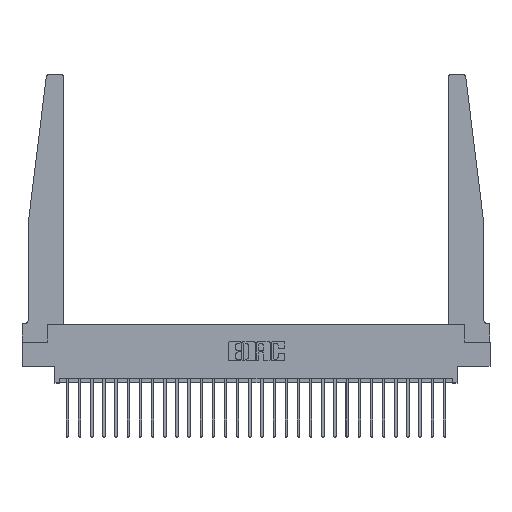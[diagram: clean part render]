
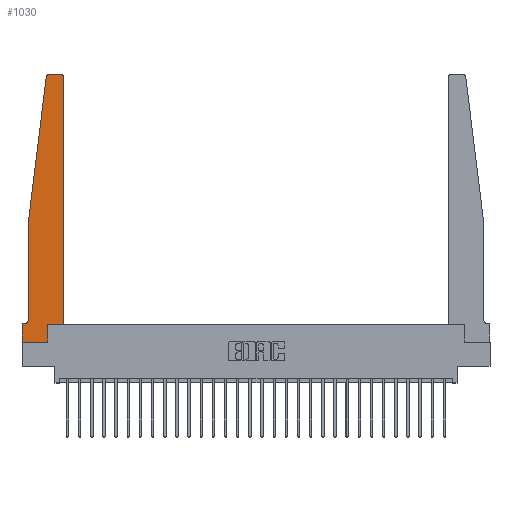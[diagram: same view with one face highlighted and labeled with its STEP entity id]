
A CAD part, top view. The second image highlights one B-rep face of the part: STEP entity #1030.
In plain terms, the highlighted planar face has unit normal (0, 0, 1).
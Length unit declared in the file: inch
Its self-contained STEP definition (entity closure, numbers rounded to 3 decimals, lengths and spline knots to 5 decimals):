
#141 = DIRECTION ( 'NONE',  ( -0.122, -0.992, 0. ) ) ;
#332 = DIRECTION ( 'NONE',  ( 1., 0., 0. ) ) ;
#891 = CARTESIAN_POINT ( 'NONE',  ( 0., 0., 0.37 ) ) ;
#1030 = ADVANCED_FACE ( 'NONE', ( #24861 ), #23354, .T. ) ;
#1106 = CIRCLE ( 'NONE', #11895, 0.03 ) ;
#1313 = VERTEX_POINT ( 'NONE', #19991 ) ;
#1432 = CARTESIAN_POINT ( 'NONE',  ( 0.2605, 0.18, 0.37 ) ) ;
#1592 = LINE ( 'NONE', #1432, #17585 ) ;
#1642 = ORIENTED_EDGE ( 'NONE', *, *, #18052, .T. ) ;
#1801 = VECTOR ( 'NONE', #141, 39.37008 ) ;
#2318 = VERTEX_POINT ( 'NONE', #25213 ) ;
#3016 = EDGE_CURVE ( 'NONE', #20631, #13860, #7359, .T. ) ;
#3051 = EDGE_CURVE ( 'NONE', #24581, #18007, #3779, .T. ) ;
#3184 = CARTESIAN_POINT ( 'NONE',  ( 0.425, 0.18, 0.37 ) ) ;
#3285 = CARTESIAN_POINT ( 'NONE',  ( 0.065, 0.2375, 0.37 ) ) ;
#3527 = CARTESIAN_POINT ( 'NONE',  ( 0.065, 1.25, 0.37 ) ) ;
#3779 = LINE ( 'NONE', #23258, #6710 ) ;
#5080 = CARTESIAN_POINT ( 'NONE',  ( 0.395, 2.72, 0.37 ) ) ;
#5650 = LINE ( 'NONE', #7865, #21712 ) ;
#6386 = CARTESIAN_POINT ( 'NONE',  ( 0.065, 1.25, 0.37 ) ) ;
#6434 = VERTEX_POINT ( 'NONE', #12352 ) ;
#6580 = CARTESIAN_POINT ( 'NONE',  ( 0.27653, 2.72, 0.37 ) ) ;
#6613 = VERTEX_POINT ( 'NONE', #9501 ) ;
#6710 = VECTOR ( 'NONE', #10661, 39.37008 ) ;
#7160 = DIRECTION ( 'NONE',  ( 1., 0., 0. ) ) ;
#7359 = LINE ( 'NONE', #6386, #1801 ) ;
#7554 = EDGE_LOOP ( 'NONE', ( #24490, #23443, #11855, #10451, #11024, #9174, #17114, #26584, #1642, #20794, #8621, #11770 ) ) ;
#7865 = CARTESIAN_POINT ( 'NONE',  ( 0.425, 0.18, 0.37 ) ) ;
#8099 = EDGE_CURVE ( 'NONE', #20376, #22676, #22496, .T. ) ;
#8511 = CARTESIAN_POINT ( 'NONE',  ( 0.015, 0.2375, 0.37 ) ) ;
#8621 = ORIENTED_EDGE ( 'NONE', *, *, #22304, .T. ) ;
#8670 = DIRECTION ( 'NONE',  ( 1., 0., 0. ) ) ;
#8781 = EDGE_CURVE ( 'NONE', #6613, #20631, #26359, .T. ) ;
#9174 = ORIENTED_EDGE ( 'NONE', *, *, #21158, .T. ) ;
#9501 = CARTESIAN_POINT ( 'NONE',  ( 0.27653, 2.75, 0.37 ) ) ;
#9759 = LINE ( 'NONE', #891, #25851 ) ;
#9957 = LINE ( 'NONE', #3527, #25399 ) ;
#9962 = DIRECTION ( 'NONE',  ( 0., 1., 0. ) ) ;
#9964 = LINE ( 'NONE', #10710, #26066 ) ;
#10451 = ORIENTED_EDGE ( 'NONE', *, *, #13457, .T. ) ;
#10615 = DIRECTION ( 'NONE',  ( -1., 0., 0. ) ) ;
#10661 = DIRECTION ( 'NONE',  ( 0., -1., 0. ) ) ;
#10710 = CARTESIAN_POINT ( 'NONE',  ( 0.25, 2.75, 0.37 ) ) ;
#11024 = ORIENTED_EDGE ( 'NONE', *, *, #8099, .T. ) ;
#11770 = ORIENTED_EDGE ( 'NONE', *, *, #13896, .T. ) ;
#11824 = DIRECTION ( 'NONE',  ( 0., -1., 0. ) ) ;
#11855 = ORIENTED_EDGE ( 'NONE', *, *, #3016, .T. ) ;
#11895 = AXIS2_PLACEMENT_3D ( 'NONE', #5080, #19681, #7160 ) ;
#12352 = CARTESIAN_POINT ( 'NONE',  ( 0.425, 0.18, 0.37 ) ) ;
#12403 = CARTESIAN_POINT ( 'NONE',  ( 0.24675, 2.72367, 0.37 ) ) ;
#12672 = DIRECTION ( 'NONE',  ( -1., 0., 0. ) ) ;
#12842 = DIRECTION ( 'NONE',  ( 0., 0., 1. ) ) ;
#13457 = EDGE_CURVE ( 'NONE', #13860, #20376, #9957, .T. ) ;
#13478 = CARTESIAN_POINT ( 'NONE',  ( 0., 0.1875, 0.37 ) ) ;
#13860 = VERTEX_POINT ( 'NONE', #17448 ) ;
#13896 = EDGE_CURVE ( 'NONE', #1313, #2318, #1106, .T. ) ;
#13939 = DIRECTION ( 'NONE',  ( 0., 1., 0. ) ) ;
#14250 = CARTESIAN_POINT ( 'NONE',  ( 0.2605, 0.18, 0.37 ) ) ;
#15019 = LINE ( 'NONE', #3184, #19298 ) ;
#15956 = EDGE_CURVE ( 'NONE', #18213, #6434, #15019, .T. ) ;
#16305 = VERTEX_POINT ( 'NONE', #23333 ) ;
#17114 = ORIENTED_EDGE ( 'NONE', *, *, #3051, .T. ) ;
#17448 = CARTESIAN_POINT ( 'NONE',  ( 0.065, 1.25, 0.37 ) ) ;
#17585 = VECTOR ( 'NONE', #13939, 39.37008 ) ;
#17590 = DIRECTION ( 'NONE',  ( 1., 0., 0. ) ) ;
#17781 = DIRECTION ( 'NONE',  ( 1., 0., 0. ) ) ;
#17893 = EDGE_CURVE ( 'NONE', #18007, #16305, #9759, .T. ) ;
#18007 = VERTEX_POINT ( 'NONE', #18041 ) ;
#18041 = CARTESIAN_POINT ( 'NONE',  ( 0., 0., 0.37 ) ) ;
#18052 = EDGE_CURVE ( 'NONE', #16305, #18213, #1592, .T. ) ;
#18213 = VERTEX_POINT ( 'NONE', #14250 ) ;
#19026 = DIRECTION ( 'NONE',  ( -1., 0., 0. ) ) ;
#19298 = VECTOR ( 'NONE', #17781, 39.37008 ) ;
#19678 = EDGE_CURVE ( 'NONE', #2318, #6613, #9964, .T. ) ;
#19681 = DIRECTION ( 'NONE',  ( 0., 0., 1. ) ) ;
#19991 = CARTESIAN_POINT ( 'NONE',  ( 0.425, 2.72, 0.37 ) ) ;
#20376 = VERTEX_POINT ( 'NONE', #3285 ) ;
#20631 = VERTEX_POINT ( 'NONE', #12403 ) ;
#20794 = ORIENTED_EDGE ( 'NONE', *, *, #15956, .T. ) ;
#21028 = CARTESIAN_POINT ( 'NONE',  ( 0.065, 0.1875, 0.37 ) ) ;
#21158 = EDGE_CURVE ( 'NONE', #22676, #24581, #26643, .T. ) ;
#21228 = DIRECTION ( 'NONE',  ( 0., 0., 1. ) ) ;
#21712 = VECTOR ( 'NONE', #9962, 39.37008 ) ;
#22304 = EDGE_CURVE ( 'NONE', #6434, #1313, #5650, .T. ) ;
#22496 = CIRCLE ( 'NONE', #26057, 0.05 ) ;
#22676 = VERTEX_POINT ( 'NONE', #23549 ) ;
#23220 = DIRECTION ( 'NONE',  ( 0., 0., -1. ) ) ;
#23258 = CARTESIAN_POINT ( 'NONE',  ( 0., 0., 0.37 ) ) ;
#23333 = CARTESIAN_POINT ( 'NONE',  ( 0.2605, 0., 0.37 ) ) ;
#23354 = PLANE ( 'NONE',  #26663 ) ;
#23443 = ORIENTED_EDGE ( 'NONE', *, *, #8781, .T. ) ;
#23549 = CARTESIAN_POINT ( 'NONE',  ( 0.015, 0.1875, 0.37 ) ) ;
#23613 = AXIS2_PLACEMENT_3D ( 'NONE', #6580, #21228, #8670 ) ;
#24490 = ORIENTED_EDGE ( 'NONE', *, *, #19678, .T. ) ;
#24581 = VERTEX_POINT ( 'NONE', #13478 ) ;
#24861 = FACE_OUTER_BOUND ( 'NONE', #7554, .T. ) ;
#25213 = CARTESIAN_POINT ( 'NONE',  ( 0.395, 2.75, 0.37 ) ) ;
#25399 = VECTOR ( 'NONE', #11824, 39.37008 ) ;
#25451 = CARTESIAN_POINT ( 'NONE',  ( 0., 0.1875, 0.37 ) ) ;
#25851 = VECTOR ( 'NONE', #17590, 39.37008 ) ;
#25985 = VECTOR ( 'NONE', #12672, 39.37008 ) ;
#26057 = AXIS2_PLACEMENT_3D ( 'NONE', #8511, #23220, #10615 ) ;
#26066 = VECTOR ( 'NONE', #19026, 39.37008 ) ;
#26359 = CIRCLE ( 'NONE', #23613, 0.03 ) ;
#26584 = ORIENTED_EDGE ( 'NONE', *, *, #17893, .T. ) ;
#26643 = LINE ( 'NONE', #21028, #25985 ) ;
#26663 = AXIS2_PLACEMENT_3D ( 'NONE', #25451, #12842, #332 ) ;
